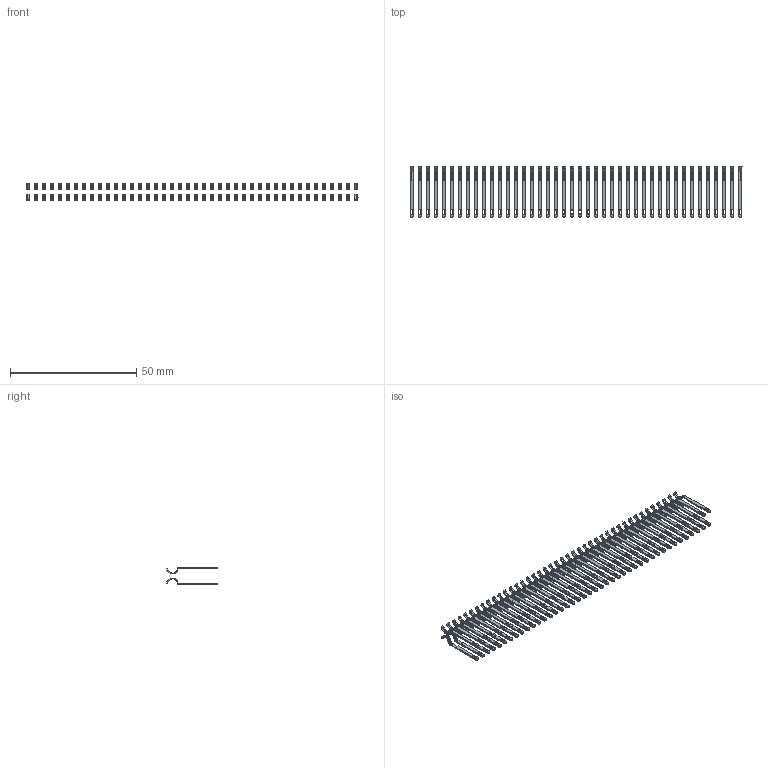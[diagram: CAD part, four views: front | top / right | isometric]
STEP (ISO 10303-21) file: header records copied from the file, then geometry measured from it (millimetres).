
FILE_DESCRIPTION (( 'STEP AP203' ), '1' );
FILE_NAME ('346-084-500-804.STEP', '2018-08-29T10:41:02', ( '' ), ( '' ), 'SwSTEP 2.0', 'SolidWorks 2016', '' );
FILE_SCHEMA (( 'CONFIG_CONTROL_DESIGN' ));
Length unit declared in the file: inch
Products named in the file (3): 346 Part_0.170 Offset - 0.156 Dia-TH; 345-292-001_345-293-100; 346-084-500-804
Assembly tree (85 placements, depth 2):
  346-084-500-804
    346 Part_0.170 Offset - 0.156 Dia-TH
    345-292-001_345-293-100  x84
Bounding box: 131.44 x 19.94 x 6.99 mm (x, y, z)
Volume: 1012.5 mm3; surface area: 6630.3 mm2
Topology: 84 solids, 84 shells, 3528 faces, 10584 edges, 7056 vertices
Faces by surface type: plane 2016, cylinder 1512
Entity records: 27475 total; most frequent: CARTESIAN_POINT 4528, ORIENTED_EDGE 4462, DIRECTION 4043, EDGE_CURVE 2231, LINE 1927, VECTOR 1927, VERTEX_POINT 1486, AXIS2_PLACEMENT_3D 1058
